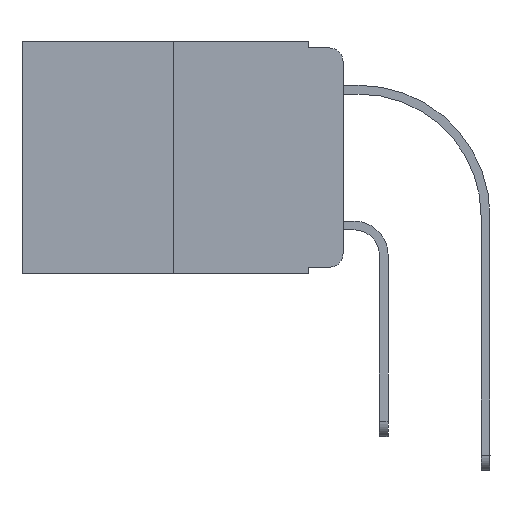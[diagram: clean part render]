
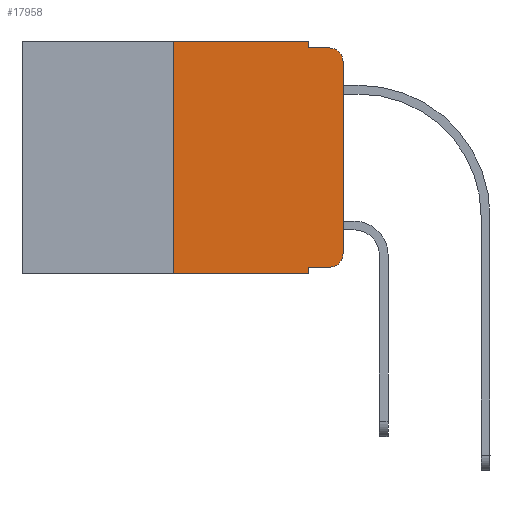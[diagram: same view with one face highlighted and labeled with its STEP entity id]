
A CAD part, left-side view. The second image highlights one B-rep face of the part: STEP entity #17958.
In plain terms, the highlighted planar face has unit normal (-1, 0, 0).
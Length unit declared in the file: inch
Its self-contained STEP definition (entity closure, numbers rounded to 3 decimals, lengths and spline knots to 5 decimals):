
#754 = VERTEX_POINT ( 'NONE', #13771 ) ;
#913 = VECTOR ( 'NONE', #16812, 39.37008 ) ;
#959 = LINE ( 'NONE', #11365, #913 ) ;
#1150 = CARTESIAN_POINT ( 'NONE',  ( 0., 0.051, -0.333 ) ) ;
#1169 = ORIENTED_EDGE ( 'NONE', *, *, #7652, .F. ) ;
#1501 = ORIENTED_EDGE ( 'NONE', *, *, #15264, .F. ) ;
#1607 = CARTESIAN_POINT ( 'NONE',  ( 0., 0.02, -0.01 ) ) ;
#1614 = DIRECTION ( 'NONE',  ( 0., 0., -1. ) ) ;
#1715 = CARTESIAN_POINT ( 'NONE',  ( 0., 0.051, 0. ) ) ;
#1937 = DIRECTION ( 'NONE',  ( 0., 0., -1. ) ) ;
#2110 = VECTOR ( 'NONE', #13285, 39.37008 ) ;
#2294 = DIRECTION ( 'NONE',  ( 1., 0., 0. ) ) ;
#2788 = DIRECTION ( 'NONE',  ( 0., 0., 1. ) ) ;
#3095 = VECTOR ( 'NONE', #13281, 39.37008 ) ;
#3659 = VERTEX_POINT ( 'NONE', #8781 ) ;
#3691 = AXIS2_PLACEMENT_3D ( 'NONE', #7852, #2294, #6158 ) ;
#3743 = EDGE_CURVE ( 'NONE', #11509, #6306, #19055, .T. ) ;
#4970 = ORIENTED_EDGE ( 'NONE', *, *, #20511, .F. ) ;
#5551 = ORIENTED_EDGE ( 'NONE', *, *, #20950, .T. ) ;
#6158 = DIRECTION ( 'NONE',  ( 0., 0., -1. ) ) ;
#6306 = VERTEX_POINT ( 'NONE', #1607 ) ;
#6375 = DIRECTION ( 'NONE',  ( 0., 0., -1. ) ) ;
#6407 = ORIENTED_EDGE ( 'NONE', *, *, #10129, .F. ) ;
#6740 = CARTESIAN_POINT ( 'NONE',  ( 0., 0.25, -0.343 ) ) ;
#7512 = PLANE ( 'NONE',  #3691 ) ;
#7652 = EDGE_CURVE ( 'NONE', #754, #11917, #9141, .T. ) ;
#7852 = CARTESIAN_POINT ( 'NONE',  ( 0., 0.473, 0. ) ) ;
#7871 = CARTESIAN_POINT ( 'NONE',  ( 0., 0.25, 0. ) ) ;
#8356 = EDGE_CURVE ( 'NONE', #14896, #11509, #11391, .T. ) ;
#8781 = CARTESIAN_POINT ( 'NONE',  ( 0., 0.02, -0.333 ) ) ;
#9103 = EDGE_CURVE ( 'NONE', #3659, #14896, #18403, .T. ) ;
#9141 = LINE ( 'NONE', #21601, #21588 ) ;
#9648 = LINE ( 'NONE', #18389, #2110 ) ;
#9672 = DIRECTION ( 'NONE',  ( 0., 0., 1. ) ) ;
#9682 = VECTOR ( 'NONE', #20601, 39.37008 ) ;
#10049 = EDGE_CURVE ( 'NONE', #17616, #12035, #21577, .T. ) ;
#10104 = CARTESIAN_POINT ( 'NONE',  ( 0., 0.02, -0.03 ) ) ;
#10129 = EDGE_CURVE ( 'NONE', #12035, #13168, #959, .T. ) ;
#10309 = LINE ( 'NONE', #1715, #19788 ) ;
#10336 = ORIENTED_EDGE ( 'NONE', *, *, #9103, .T. ) ;
#10461 = CARTESIAN_POINT ( 'NONE',  ( 0., 0.02, -0.313 ) ) ;
#10510 = LINE ( 'NONE', #11986, #9682 ) ;
#10551 = ORIENTED_EDGE ( 'NONE', *, *, #10049, .F. ) ;
#10679 = VECTOR ( 'NONE', #9672, 39.37008 ) ;
#11275 = DIRECTION ( 'NONE',  ( 0., 0., -1. ) ) ;
#11365 = CARTESIAN_POINT ( 'NONE',  ( 0., 0.473, 0. ) ) ;
#11391 = LINE ( 'NONE', #19893, #19729 ) ;
#11509 = VERTEX_POINT ( 'NONE', #20012 ) ;
#11797 = CARTESIAN_POINT ( 'NONE',  ( 0., 0.051, -0.343 ) ) ;
#11917 = VERTEX_POINT ( 'NONE', #11797 ) ;
#11955 = EDGE_CURVE ( 'NONE', #754, #3659, #13392, .T. ) ;
#11986 = CARTESIAN_POINT ( 'NONE',  ( 0., 0.473, -0.343 ) ) ;
#12035 = VERTEX_POINT ( 'NONE', #14734 ) ;
#12037 = DIRECTION ( 'NONE',  ( -1., 0., 0. ) ) ;
#12714 = ORIENTED_EDGE ( 'NONE', *, *, #11955, .T. ) ;
#13086 = CARTESIAN_POINT ( 'NONE',  ( 0., 0., -0.313 ) ) ;
#13111 = CARTESIAN_POINT ( 'NONE',  ( 0., 0.051, 0. ) ) ;
#13168 = VERTEX_POINT ( 'NONE', #13111 ) ;
#13281 = DIRECTION ( 'NONE',  ( 0., -1., 0. ) ) ;
#13285 = DIRECTION ( 'NONE',  ( 0., -1., 0. ) ) ;
#13313 = CARTESIAN_POINT ( 'NONE',  ( 0., 0.051, -0.01 ) ) ;
#13392 = LINE ( 'NONE', #1150, #3095 ) ;
#13771 = CARTESIAN_POINT ( 'NONE',  ( 0., 0.051, -0.333 ) ) ;
#14734 = CARTESIAN_POINT ( 'NONE',  ( 0., 0.25, 0. ) ) ;
#14896 = VERTEX_POINT ( 'NONE', #13086 ) ;
#15264 = EDGE_CURVE ( 'NONE', #21735, #6306, #9648, .T. ) ;
#16812 = DIRECTION ( 'NONE',  ( 0., -1., 0. ) ) ;
#17616 = VERTEX_POINT ( 'NONE', #6740 ) ;
#17689 = AXIS2_PLACEMENT_3D ( 'NONE', #10461, #12037, #1614 ) ;
#17958 = ADVANCED_FACE ( 'NONE', ( #19519 ), #7512, .F. ) ;
#17979 = AXIS2_PLACEMENT_3D ( 'NONE', #10104, #21774, #6375 ) ;
#18389 = CARTESIAN_POINT ( 'NONE',  ( 0., 0.051, -0.01 ) ) ;
#18403 = CIRCLE ( 'NONE', #17689, 0.02 ) ;
#19055 = CIRCLE ( 'NONE', #17979, 0.02 ) ;
#19519 = FACE_OUTER_BOUND ( 'NONE', #21862, .T. ) ;
#19729 = VECTOR ( 'NONE', #2788, 39.37008 ) ;
#19788 = VECTOR ( 'NONE', #1937, 39.37008 ) ;
#19893 = CARTESIAN_POINT ( 'NONE',  ( 0., 0., 0. ) ) ;
#20012 = CARTESIAN_POINT ( 'NONE',  ( 0., 0., -0.03 ) ) ;
#20159 = ORIENTED_EDGE ( 'NONE', *, *, #8356, .T. ) ;
#20511 = EDGE_CURVE ( 'NONE', #13168, #21735, #10309, .T. ) ;
#20601 = DIRECTION ( 'NONE',  ( 0., -1., 0. ) ) ;
#20950 = EDGE_CURVE ( 'NONE', #17616, #11917, #10510, .T. ) ;
#21577 = LINE ( 'NONE', #7871, #10679 ) ;
#21588 = VECTOR ( 'NONE', #11275, 39.37008 ) ;
#21601 = CARTESIAN_POINT ( 'NONE',  ( 0., 0.051, 0. ) ) ;
#21735 = VERTEX_POINT ( 'NONE', #13313 ) ;
#21774 = DIRECTION ( 'NONE',  ( -1., 0., 0. ) ) ;
#21862 = EDGE_LOOP ( 'NONE', ( #20159, #22175, #1501, #4970, #6407, #10551, #5551, #1169, #12714, #10336 ) ) ;
#22175 = ORIENTED_EDGE ( 'NONE', *, *, #3743, .T. ) ;
